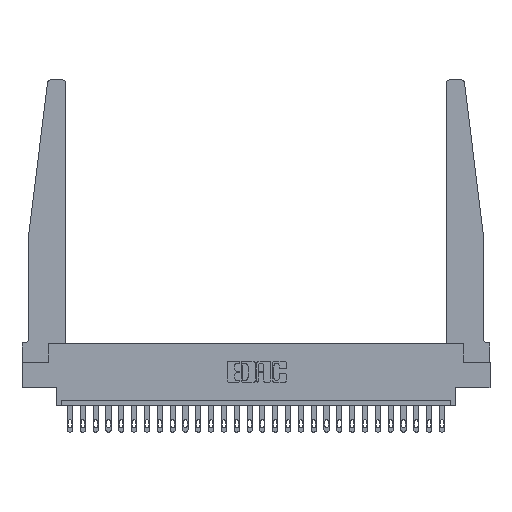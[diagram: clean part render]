
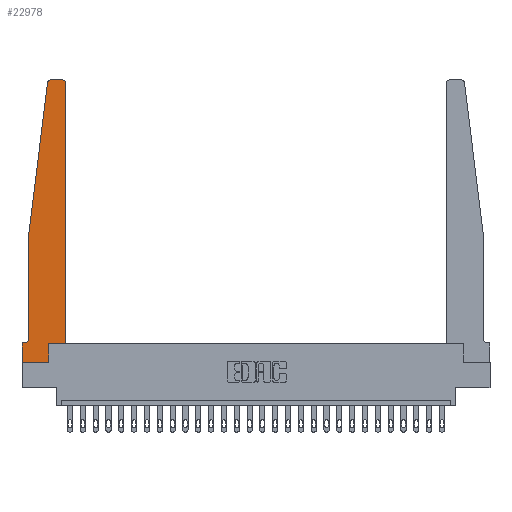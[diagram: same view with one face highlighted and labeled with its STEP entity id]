
A CAD part, top view. The second image highlights one B-rep face of the part: STEP entity #22978.
In plain terms, the highlighted planar face has unit normal (0, 0, 1).
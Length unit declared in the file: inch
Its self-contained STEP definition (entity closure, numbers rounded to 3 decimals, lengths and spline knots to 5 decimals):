
#75 = CARTESIAN_POINT ( 'NONE',  ( 0., 0., 0.37 ) ) ;
#365 = CARTESIAN_POINT ( 'NONE',  ( 0.2605, 0.18, 0.37 ) ) ;
#701 = DIRECTION ( 'NONE',  ( -1., 0., 0. ) ) ;
#1196 = CARTESIAN_POINT ( 'NONE',  ( 0.24675, 2.72367, 0.37 ) ) ;
#1356 = VERTEX_POINT ( 'NONE', #24846 ) ;
#1365 = ORIENTED_EDGE ( 'NONE', *, *, #23572, .T. ) ;
#1403 = EDGE_CURVE ( 'NONE', #21560, #14656, #5723, .T. ) ;
#1810 = CARTESIAN_POINT ( 'NONE',  ( 0., 0., 0.37 ) ) ;
#1847 = ORIENTED_EDGE ( 'NONE', *, *, #20234, .T. ) ;
#2265 = LINE ( 'NONE', #8201, #10243 ) ;
#2304 = CARTESIAN_POINT ( 'NONE',  ( 0.2605, 0.18, 0.37 ) ) ;
#2965 = CARTESIAN_POINT ( 'NONE',  ( 0.425, 0.18, 0.37 ) ) ;
#3567 = DIRECTION ( 'NONE',  ( -1., 0., 0. ) ) ;
#3751 = PLANE ( 'NONE',  #20136 ) ;
#3783 = DIRECTION ( 'NONE',  ( 1., 0., 0. ) ) ;
#4001 = VECTOR ( 'NONE', #10038, 39.37008 ) ;
#4276 = VERTEX_POINT ( 'NONE', #17769 ) ;
#4460 = AXIS2_PLACEMENT_3D ( 'NONE', #25464, #15406, #3783 ) ;
#4518 = LINE ( 'NONE', #2965, #18453 ) ;
#5117 = ORIENTED_EDGE ( 'NONE', *, *, #12201, .T. ) ;
#5318 = VECTOR ( 'NONE', #20088, 39.37008 ) ;
#5723 = LINE ( 'NONE', #13611, #12016 ) ;
#6005 = ORIENTED_EDGE ( 'NONE', *, *, #21649, .T. ) ;
#6083 = VERTEX_POINT ( 'NONE', #24593 ) ;
#6434 = CARTESIAN_POINT ( 'NONE',  ( 0.015, 0.1875, 0.37 ) ) ;
#6485 = VECTOR ( 'NONE', #23799, 39.37008 ) ;
#6730 = DIRECTION ( 'NONE',  ( 0., 0., 1. ) ) ;
#8201 = CARTESIAN_POINT ( 'NONE',  ( 0.065, 1.25, 0.37 ) ) ;
#8240 = CARTESIAN_POINT ( 'NONE',  ( 0.065, 0.1875, 0.37 ) ) ;
#8375 = LINE ( 'NONE', #8240, #5318 ) ;
#8394 = DIRECTION ( 'NONE',  ( 1., 0., 0. ) ) ;
#8436 = CARTESIAN_POINT ( 'NONE',  ( 0.065, 1.25, 0.37 ) ) ;
#8830 = EDGE_CURVE ( 'NONE', #6083, #23099, #9743, .T. ) ;
#9384 = CARTESIAN_POINT ( 'NONE',  ( 0.25, 2.75, 0.37 ) ) ;
#9392 = VECTOR ( 'NONE', #8394, 39.37008 ) ;
#9437 = DIRECTION ( 'NONE',  ( 0., 0., 1. ) ) ;
#9743 = CIRCLE ( 'NONE', #21696, 0.05 ) ;
#10038 = DIRECTION ( 'NONE',  ( 0., 1., 0. ) ) ;
#10243 = VECTOR ( 'NONE', #18233, 39.37008 ) ;
#10503 = DIRECTION ( 'NONE',  ( 0., 0., -1. ) ) ;
#10611 = ORIENTED_EDGE ( 'NONE', *, *, #22291, .T. ) ;
#10641 = EDGE_CURVE ( 'NONE', #23295, #4276, #18850, .T. ) ;
#10694 = ORIENTED_EDGE ( 'NONE', *, *, #16989, .T. ) ;
#11208 = LINE ( 'NONE', #9384, #19370 ) ;
#11255 = FACE_OUTER_BOUND ( 'NONE', #21973, .T. ) ;
#11642 = CARTESIAN_POINT ( 'NONE',  ( 0., 0.1875, 0.37 ) ) ;
#12016 = VECTOR ( 'NONE', #25229, 39.37008 ) ;
#12038 = CARTESIAN_POINT ( 'NONE',  ( 0.2605, 0., 0.37 ) ) ;
#12201 = EDGE_CURVE ( 'NONE', #1356, #23295, #4518, .T. ) ;
#12668 = ORIENTED_EDGE ( 'NONE', *, *, #1403, .T. ) ;
#13611 = CARTESIAN_POINT ( 'NONE',  ( 0., 0., 0.37 ) ) ;
#14186 = CARTESIAN_POINT ( 'NONE',  ( 0.425, 0.18, 0.37 ) ) ;
#14656 = VERTEX_POINT ( 'NONE', #12038 ) ;
#14838 = DIRECTION ( 'NONE',  ( 0., 1., 0. ) ) ;
#15021 = EDGE_CURVE ( 'NONE', #14656, #24959, #20332, .T. ) ;
#15400 = EDGE_CURVE ( 'NONE', #20908, #21560, #15796, .T. ) ;
#15406 = DIRECTION ( 'NONE',  ( 0., 0., 1. ) ) ;
#15581 = AXIS2_PLACEMENT_3D ( 'NONE', #20670, #6730, #20156 ) ;
#15796 = LINE ( 'NONE', #75, #6485 ) ;
#16104 = ORIENTED_EDGE ( 'NONE', *, *, #15400, .T. ) ;
#16989 = EDGE_CURVE ( 'NONE', #24010, #6083, #23009, .T. ) ;
#17692 = DIRECTION ( 'NONE',  ( 0., -1., 0. ) ) ;
#17769 = CARTESIAN_POINT ( 'NONE',  ( 0.395, 2.75, 0.37 ) ) ;
#18100 = CARTESIAN_POINT ( 'NONE',  ( 0.015, 0.2375, 0.37 ) ) ;
#18233 = DIRECTION ( 'NONE',  ( -0.122, -0.992, 0. ) ) ;
#18453 = VECTOR ( 'NONE', #14838, 39.37008 ) ;
#18712 = ORIENTED_EDGE ( 'NONE', *, *, #10641, .T. ) ;
#18850 = CIRCLE ( 'NONE', #15581, 0.03 ) ;
#19095 = CARTESIAN_POINT ( 'NONE',  ( 0.27653, 2.75, 0.37 ) ) ;
#19370 = VECTOR ( 'NONE', #3567, 39.37008 ) ;
#19482 = DIRECTION ( 'NONE',  ( 1., 0., 0. ) ) ;
#19857 = VERTEX_POINT ( 'NONE', #19095 ) ;
#20088 = DIRECTION ( 'NONE',  ( -1., 0., 0. ) ) ;
#20136 = AXIS2_PLACEMENT_3D ( 'NONE', #11642, #9437, #19482 ) ;
#20156 = DIRECTION ( 'NONE',  ( 1., 0., 0. ) ) ;
#20234 = EDGE_CURVE ( 'NONE', #4276, #19857, #11208, .T. ) ;
#20332 = LINE ( 'NONE', #365, #4001 ) ;
#20670 = CARTESIAN_POINT ( 'NONE',  ( 0.395, 2.72, 0.37 ) ) ;
#20801 = ORIENTED_EDGE ( 'NONE', *, *, #8830, .T. ) ;
#20908 = VERTEX_POINT ( 'NONE', #22500 ) ;
#21235 = ORIENTED_EDGE ( 'NONE', *, *, #15021, .T. ) ;
#21560 = VERTEX_POINT ( 'NONE', #1810 ) ;
#21578 = CARTESIAN_POINT ( 'NONE',  ( 0.065, 1.25, 0.37 ) ) ;
#21649 = EDGE_CURVE ( 'NONE', #24959, #1356, #22185, .T. ) ;
#21696 = AXIS2_PLACEMENT_3D ( 'NONE', #18100, #10503, #701 ) ;
#21973 = EDGE_LOOP ( 'NONE', ( #1847, #22188, #10611, #10694, #20801, #1365, #16104, #12668, #21235, #6005, #5117, #18712 ) ) ;
#22185 = LINE ( 'NONE', #14186, #9392 ) ;
#22188 = ORIENTED_EDGE ( 'NONE', *, *, #22511, .T. ) ;
#22291 = EDGE_CURVE ( 'NONE', #22836, #24010, #2265, .T. ) ;
#22500 = CARTESIAN_POINT ( 'NONE',  ( 0., 0.1875, 0.37 ) ) ;
#22511 = EDGE_CURVE ( 'NONE', #19857, #22836, #25076, .T. ) ;
#22584 = VECTOR ( 'NONE', #17692, 39.37008 ) ;
#22825 = CARTESIAN_POINT ( 'NONE',  ( 0.425, 2.72, 0.37 ) ) ;
#22836 = VERTEX_POINT ( 'NONE', #1196 ) ;
#22978 = ADVANCED_FACE ( 'NONE', ( #11255 ), #3751, .T. ) ;
#23009 = LINE ( 'NONE', #21578, #22584 ) ;
#23099 = VERTEX_POINT ( 'NONE', #6434 ) ;
#23295 = VERTEX_POINT ( 'NONE', #22825 ) ;
#23572 = EDGE_CURVE ( 'NONE', #23099, #20908, #8375, .T. ) ;
#23799 = DIRECTION ( 'NONE',  ( 0., -1., 0. ) ) ;
#24010 = VERTEX_POINT ( 'NONE', #8436 ) ;
#24593 = CARTESIAN_POINT ( 'NONE',  ( 0.065, 0.2375, 0.37 ) ) ;
#24846 = CARTESIAN_POINT ( 'NONE',  ( 0.425, 0.18, 0.37 ) ) ;
#24959 = VERTEX_POINT ( 'NONE', #2304 ) ;
#25076 = CIRCLE ( 'NONE', #4460, 0.03 ) ;
#25229 = DIRECTION ( 'NONE',  ( 1., 0., 0. ) ) ;
#25464 = CARTESIAN_POINT ( 'NONE',  ( 0.27653, 2.72, 0.37 ) ) ;
